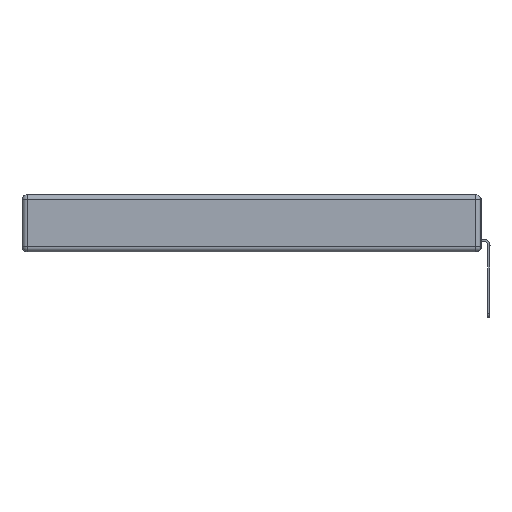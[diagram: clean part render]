
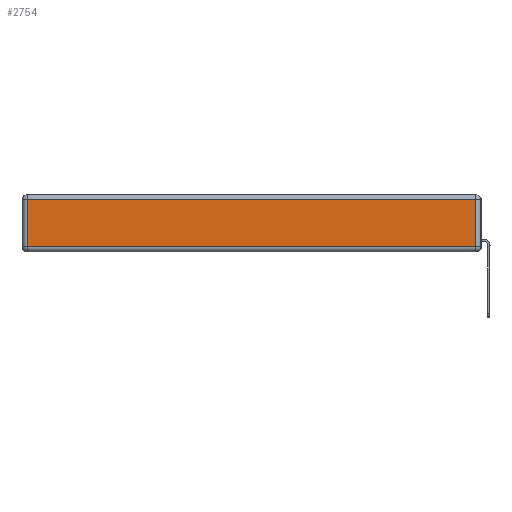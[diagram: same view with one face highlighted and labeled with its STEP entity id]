
A CAD part, left-side view. The second image highlights one B-rep face of the part: STEP entity #2754.
In plain terms, the highlighted planar face has unit normal (-1, 0, 0).
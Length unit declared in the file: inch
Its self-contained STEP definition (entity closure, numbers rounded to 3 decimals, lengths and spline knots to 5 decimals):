
#780 = ORIENTED_EDGE ( 'NONE', *, *, #9892, .T. ) ;
#1244 = LINE ( 'NONE', #11958, #15002 ) ;
#1792 = EDGE_CURVE ( 'NONE', #6800, #4794, #1244, .T. ) ;
#2371 = DIRECTION ( 'NONE',  ( 0., -1., 0. ) ) ;
#2388 = LINE ( 'NONE', #7105, #15213 ) ;
#2466 = ORIENTED_EDGE ( 'NONE', *, *, #14724, .T. ) ;
#2611 = VECTOR ( 'NONE', #5858, 39.37008 ) ;
#2700 = AXIS2_PLACEMENT_3D ( 'NONE', #3238, #14054, #13894 ) ;
#2754 = ADVANCED_FACE ( 'NONE', ( #5668 ), #9318, .T. ) ;
#3238 = CARTESIAN_POINT ( 'NONE',  ( 0., 0., -0.343 ) ) ;
#4768 = CARTESIAN_POINT ( 'NONE',  ( 0., 0.03, -0.03 ) ) ;
#4794 = VERTEX_POINT ( 'NONE', #4768 ) ;
#5313 = LINE ( 'NONE', #14338, #7726 ) ;
#5390 = CARTESIAN_POINT ( 'NONE',  ( 0., 2.72, -0.313 ) ) ;
#5583 = LINE ( 'NONE', #7092, #2611 ) ;
#5668 = FACE_OUTER_BOUND ( 'NONE', #13593, .T. ) ;
#5858 = DIRECTION ( 'NONE',  ( 0., 0., -1. ) ) ;
#6706 = EDGE_CURVE ( 'NONE', #7078, #8452, #5583, .T. ) ;
#6800 = VERTEX_POINT ( 'NONE', #9632 ) ;
#7078 = VERTEX_POINT ( 'NONE', #10253 ) ;
#7092 = CARTESIAN_POINT ( 'NONE',  ( 0., 2.72, -0.343 ) ) ;
#7105 = CARTESIAN_POINT ( 'NONE',  ( 0., 0., -0.313 ) ) ;
#7726 = VECTOR ( 'NONE', #11943, 39.37008 ) ;
#7956 = ORIENTED_EDGE ( 'NONE', *, *, #1792, .T. ) ;
#8129 = ORIENTED_EDGE ( 'NONE', *, *, #6706, .T. ) ;
#8452 = VERTEX_POINT ( 'NONE', #5390 ) ;
#9318 = PLANE ( 'NONE',  #2700 ) ;
#9632 = CARTESIAN_POINT ( 'NONE',  ( 0., 0.03, -0.313 ) ) ;
#9892 = EDGE_CURVE ( 'NONE', #4794, #7078, #5313, .T. ) ;
#10253 = CARTESIAN_POINT ( 'NONE',  ( 0., 2.72, -0.03 ) ) ;
#11943 = DIRECTION ( 'NONE',  ( 0., 1., 0. ) ) ;
#11958 = CARTESIAN_POINT ( 'NONE',  ( 0., 0.03, -0.343 ) ) ;
#13163 = DIRECTION ( 'NONE',  ( 0., 0., 1. ) ) ;
#13593 = EDGE_LOOP ( 'NONE', ( #2466, #7956, #780, #8129 ) ) ;
#13894 = DIRECTION ( 'NONE',  ( 0., 0., 1. ) ) ;
#14054 = DIRECTION ( 'NONE',  ( -1., 0., 0. ) ) ;
#14338 = CARTESIAN_POINT ( 'NONE',  ( 0., 2.75, -0.03 ) ) ;
#14724 = EDGE_CURVE ( 'NONE', #8452, #6800, #2388, .T. ) ;
#15002 = VECTOR ( 'NONE', #13163, 39.37008 ) ;
#15213 = VECTOR ( 'NONE', #2371, 39.37008 ) ;
